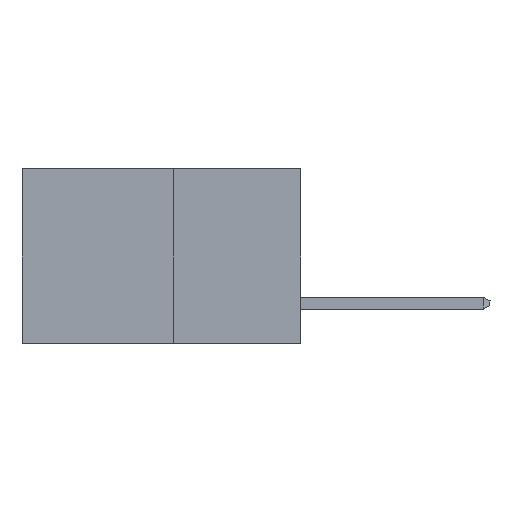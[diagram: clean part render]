
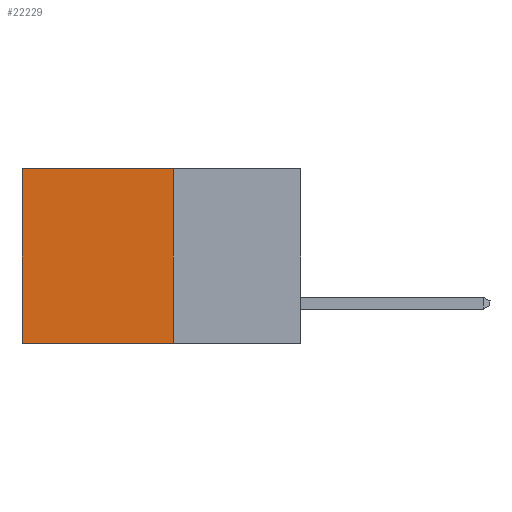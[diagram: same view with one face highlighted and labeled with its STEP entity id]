
A CAD part, left-side view. The second image highlights one B-rep face of the part: STEP entity #22229.
In plain terms, the highlighted planar face has unit normal (-1, 0, 0).
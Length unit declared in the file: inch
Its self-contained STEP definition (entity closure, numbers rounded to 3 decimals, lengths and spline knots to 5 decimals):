
#607 = VERTEX_POINT ( 'NONE', #8238 ) ;
#886 = DIRECTION ( 'NONE',  ( 0., 0., -1. ) ) ;
#2584 = EDGE_CURVE ( 'NONE', #21396, #25388, #11472, .T. ) ;
#2999 = CARTESIAN_POINT ( 'NONE',  ( 0.277, 0.59, -0.37 ) ) ;
#3024 = DIRECTION ( 'NONE',  ( 0., 0., -1. ) ) ;
#4483 = VECTOR ( 'NONE', #22956, 39.37008 ) ;
#4595 = DIRECTION ( 'NONE',  ( 1., 0., 0. ) ) ;
#4916 = VECTOR ( 'NONE', #886, 39.37008 ) ;
#6247 = CARTESIAN_POINT ( 'NONE',  ( 0.277, 0.27, 0. ) ) ;
#7485 = LINE ( 'NONE', #8385, #4483 ) ;
#8238 = CARTESIAN_POINT ( 'NONE',  ( 0.277, 0.59, 0. ) ) ;
#8249 = EDGE_CURVE ( 'NONE', #607, #25388, #16132, .T. ) ;
#8385 = CARTESIAN_POINT ( 'NONE',  ( 0.277, 0.27, 0. ) ) ;
#9911 = LINE ( 'NONE', #11437, #4916 ) ;
#9967 = ORIENTED_EDGE ( 'NONE', *, *, #20473, .T. ) ;
#10292 = ORIENTED_EDGE ( 'NONE', *, *, #2584, .F. ) ;
#10942 = DIRECTION ( 'NONE',  ( 0., 1., 0. ) ) ;
#11437 = CARTESIAN_POINT ( 'NONE',  ( 0.277, 0.27, -0.37 ) ) ;
#11472 = LINE ( 'NONE', #18565, #21868 ) ;
#14534 = ORIENTED_EDGE ( 'NONE', *, *, #8249, .T. ) ;
#15500 = VECTOR ( 'NONE', #3024, 39.37008 ) ;
#16003 = EDGE_LOOP ( 'NONE', ( #14534, #10292, #19744, #9967 ) ) ;
#16132 = LINE ( 'NONE', #2999, #15500 ) ;
#16878 = VERTEX_POINT ( 'NONE', #6247 ) ;
#17175 = PLANE ( 'NONE',  #20034 ) ;
#17198 = FACE_OUTER_BOUND ( 'NONE', #16003, .T. ) ;
#18565 = CARTESIAN_POINT ( 'NONE',  ( 0.277, 0.27, -0.37 ) ) ;
#19277 = DIRECTION ( 'NONE',  ( 0., 0., -1. ) ) ;
#19744 = ORIENTED_EDGE ( 'NONE', *, *, #25444, .F. ) ;
#20034 = AXIS2_PLACEMENT_3D ( 'NONE', #21194, #4595, #19277 ) ;
#20473 = EDGE_CURVE ( 'NONE', #16878, #607, #7485, .T. ) ;
#21194 = CARTESIAN_POINT ( 'NONE',  ( 0.277, 0.27, -0.37 ) ) ;
#21396 = VERTEX_POINT ( 'NONE', #24821 ) ;
#21696 = CARTESIAN_POINT ( 'NONE',  ( 0.277, 0.59, -0.37 ) ) ;
#21868 = VECTOR ( 'NONE', #10942, 39.37008 ) ;
#22229 = ADVANCED_FACE ( 'NONE', ( #17198 ), #17175, .F. ) ;
#22956 = DIRECTION ( 'NONE',  ( 0., 1., 0. ) ) ;
#24821 = CARTESIAN_POINT ( 'NONE',  ( 0.277, 0.27, -0.37 ) ) ;
#25388 = VERTEX_POINT ( 'NONE', #21696 ) ;
#25444 = EDGE_CURVE ( 'NONE', #16878, #21396, #9911, .T. ) ;
